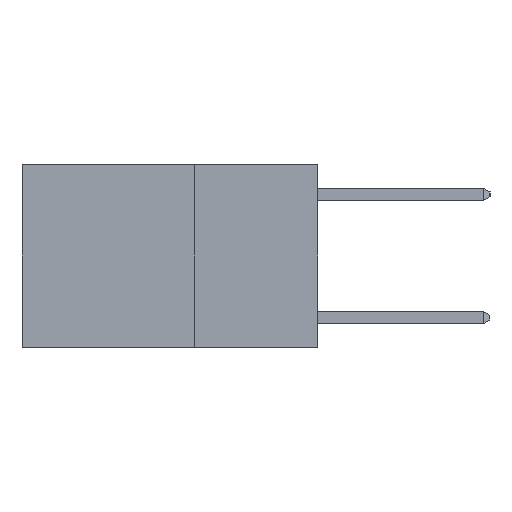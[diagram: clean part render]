
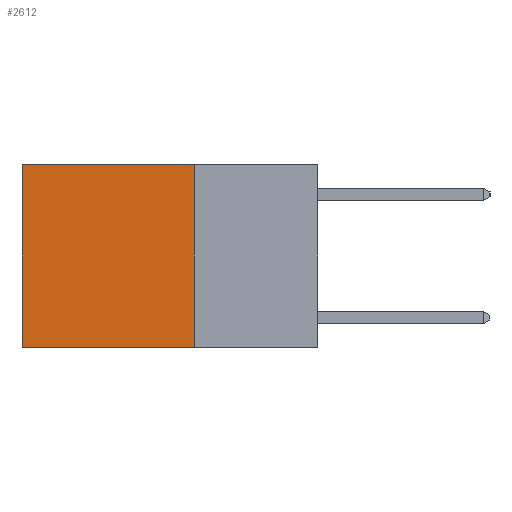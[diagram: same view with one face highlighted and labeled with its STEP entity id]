
A CAD part, left-side view. The second image highlights one B-rep face of the part: STEP entity #2612.
In plain terms, the highlighted planar face has unit normal (-1, 0, 0).
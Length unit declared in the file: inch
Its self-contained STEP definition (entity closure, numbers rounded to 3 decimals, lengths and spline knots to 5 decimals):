
#18 = CARTESIAN_POINT ( 'NONE',  ( 0.2625, 0.25, 0. ) ) ;
#143 = EDGE_LOOP ( 'NONE', ( #10318, #4866, #10855, #9753 ) ) ;
#1672 = CARTESIAN_POINT ( 'NONE',  ( 0.2625, 0.25, -0.37 ) ) ;
#1807 = FACE_OUTER_BOUND ( 'NONE', #143, .T. ) ;
#2042 = LINE ( 'NONE', #5263, #11191 ) ;
#2225 = PLANE ( 'NONE',  #4035 ) ;
#2612 = ADVANCED_FACE ( 'NONE', ( #1807 ), #2225, .F. ) ;
#2780 = VECTOR ( 'NONE', #8602, 39.37008 ) ;
#3142 = CARTESIAN_POINT ( 'NONE',  ( 0.2625, 0.25, 0. ) ) ;
#3915 = DIRECTION ( 'NONE',  ( 0., 1., 0. ) ) ;
#4035 = AXIS2_PLACEMENT_3D ( 'NONE', #3142, #9763, #4118 ) ;
#4118 = DIRECTION ( 'NONE',  ( 0., 0., -1. ) ) ;
#4824 = DIRECTION ( 'NONE',  ( 0., 0., -1. ) ) ;
#4866 = ORIENTED_EDGE ( 'NONE', *, *, #7955, .F. ) ;
#5263 = CARTESIAN_POINT ( 'NONE',  ( 0.2625, 0.25, 0. ) ) ;
#5357 = VERTEX_POINT ( 'NONE', #9254 ) ;
#5386 = CARTESIAN_POINT ( 'NONE',  ( 0.2625, 0.25, 0. ) ) ;
#5843 = CARTESIAN_POINT ( 'NONE',  ( 0.2625, 0.25, -0.37 ) ) ;
#6328 = EDGE_CURVE ( 'NONE', #8329, #7202, #2042, .T. ) ;
#6512 = CARTESIAN_POINT ( 'NONE',  ( 0.2625, 0.6, 0. ) ) ;
#6704 = EDGE_CURVE ( 'NONE', #8329, #8367, #11724, .T. ) ;
#6837 = VECTOR ( 'NONE', #4824, 39.37008 ) ;
#7202 = VERTEX_POINT ( 'NONE', #6512 ) ;
#7654 = CARTESIAN_POINT ( 'NONE',  ( 0.2625, 0.6, 0. ) ) ;
#7955 = EDGE_CURVE ( 'NONE', #8367, #5357, #9672, .T. ) ;
#8189 = DIRECTION ( 'NONE',  ( 0., 1., 0. ) ) ;
#8211 = LINE ( 'NONE', #7654, #2780 ) ;
#8329 = VERTEX_POINT ( 'NONE', #5386 ) ;
#8367 = VERTEX_POINT ( 'NONE', #1672 ) ;
#8602 = DIRECTION ( 'NONE',  ( 0., 0., -1. ) ) ;
#9254 = CARTESIAN_POINT ( 'NONE',  ( 0.2625, 0.6, -0.37 ) ) ;
#9672 = LINE ( 'NONE', #5843, #11843 ) ;
#9753 = ORIENTED_EDGE ( 'NONE', *, *, #6328, .T. ) ;
#9763 = DIRECTION ( 'NONE',  ( 1., 0., 0. ) ) ;
#10022 = EDGE_CURVE ( 'NONE', #7202, #5357, #8211, .T. ) ;
#10318 = ORIENTED_EDGE ( 'NONE', *, *, #10022, .T. ) ;
#10855 = ORIENTED_EDGE ( 'NONE', *, *, #6704, .F. ) ;
#11191 = VECTOR ( 'NONE', #8189, 39.37008 ) ;
#11724 = LINE ( 'NONE', #18, #6837 ) ;
#11843 = VECTOR ( 'NONE', #3915, 39.37008 ) ;
